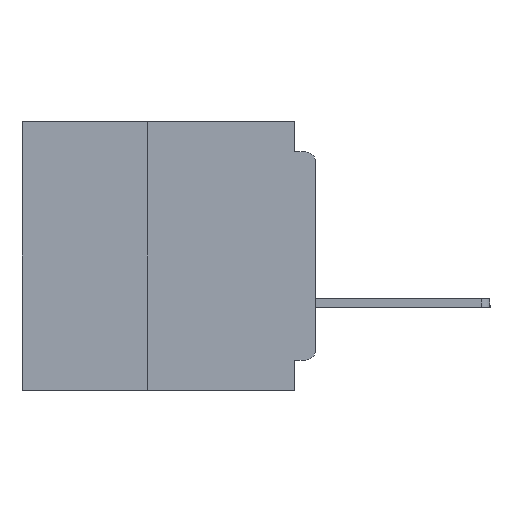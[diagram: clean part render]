
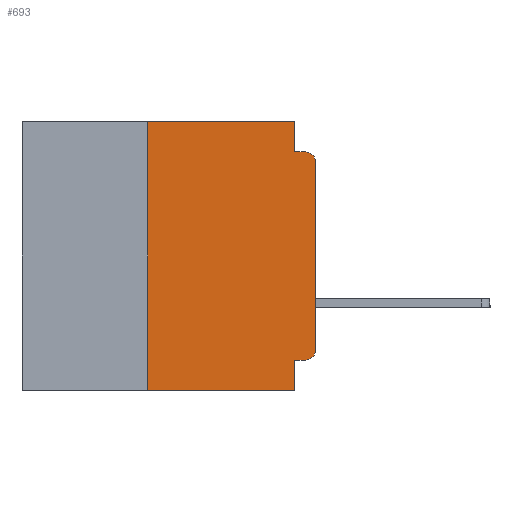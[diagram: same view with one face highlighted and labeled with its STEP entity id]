
A CAD part, left-side view. The second image highlights one B-rep face of the part: STEP entity #693.
In plain terms, the highlighted planar face has unit normal (-1, 0, 0).
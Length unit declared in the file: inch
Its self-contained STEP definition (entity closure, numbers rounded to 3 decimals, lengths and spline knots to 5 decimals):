
#657 = VERTEX_POINT ( 'NONE', #3051 ) ;
#693 = ADVANCED_FACE ( 'NONE', ( #32151 ), #5395, .F. ) ;
#718 = CARTESIAN_POINT ( 'NONE',  ( 0., 0.031, -0.045 ) ) ;
#1329 = DIRECTION ( 'NONE',  ( 0., -1., 0. ) ) ;
#1890 = CARTESIAN_POINT ( 'NONE',  ( 0., 0., -0.355 ) ) ;
#2554 = CARTESIAN_POINT ( 'NONE',  ( 0., 0.015, -0.355 ) ) ;
#3051 = CARTESIAN_POINT ( 'NONE',  ( 0., 0., -0.06 ) ) ;
#3372 = AXIS2_PLACEMENT_3D ( 'NONE', #11242, #6057, #5957 ) ;
#4143 = CARTESIAN_POINT ( 'NONE',  ( 0., 0.031, -0.4 ) ) ;
#4748 = DIRECTION ( 'NONE',  ( 0., -1., 0. ) ) ;
#4871 = VECTOR ( 'NONE', #12030, 39.37008 ) ;
#5310 = EDGE_LOOP ( 'NONE', ( #17593, #26373, #27103, #8839, #28532, #6120, #42472, #32633, #36755, #35333 ) ) ;
#5320 = DIRECTION ( 'NONE',  ( 0., 1., 0. ) ) ;
#5395 = PLANE ( 'NONE',  #3372 ) ;
#5957 = DIRECTION ( 'NONE',  ( 0., 0., -1. ) ) ;
#6057 = DIRECTION ( 'NONE',  ( 1., 0., 0. ) ) ;
#6120 = ORIENTED_EDGE ( 'NONE', *, *, #15140, .F. ) ;
#6469 = CARTESIAN_POINT ( 'NONE',  ( 0., 0.031, 0. ) ) ;
#6547 = VERTEX_POINT ( 'NONE', #18486 ) ;
#6554 = DIRECTION ( 'NONE',  ( 0., -1., 0. ) ) ;
#8559 = EDGE_CURVE ( 'NONE', #16307, #34333, #42617, .T. ) ;
#8569 = CARTESIAN_POINT ( 'NONE',  ( 0., 0.031, 0. ) ) ;
#8839 = ORIENTED_EDGE ( 'NONE', *, *, #38920, .F. ) ;
#9049 = DIRECTION ( 'NONE',  ( -1., 0., 0. ) ) ;
#9460 = VERTEX_POINT ( 'NONE', #6469 ) ;
#10446 = AXIS2_PLACEMENT_3D ( 'NONE', #29039, #9049, #32432 ) ;
#10729 = LINE ( 'NONE', #41371, #36214 ) ;
#11242 = CARTESIAN_POINT ( 'NONE',  ( 0., 0.437, 0. ) ) ;
#12005 = LINE ( 'NONE', #43093, #37463 ) ;
#12030 = DIRECTION ( 'NONE',  ( 0., 0., -1. ) ) ;
#13541 = DIRECTION ( 'NONE',  ( 0., 0., 1. ) ) ;
#13799 = LINE ( 'NONE', #14898, #21631 ) ;
#14363 = VERTEX_POINT ( 'NONE', #30455 ) ;
#14898 = CARTESIAN_POINT ( 'NONE',  ( 0., 0.437, 0. ) ) ;
#15065 = CIRCLE ( 'NONE', #33248, 0.015 ) ;
#15140 = EDGE_CURVE ( 'NONE', #6547, #39524, #37476, .T. ) ;
#16307 = VERTEX_POINT ( 'NONE', #2554 ) ;
#17262 = VERTEX_POINT ( 'NONE', #40918 ) ;
#17593 = ORIENTED_EDGE ( 'NONE', *, *, #25316, .T. ) ;
#18357 = CARTESIAN_POINT ( 'NONE',  ( 0., 0.25, -0.4 ) ) ;
#18486 = CARTESIAN_POINT ( 'NONE',  ( 0., 0.25, -0.4 ) ) ;
#18501 = EDGE_CURVE ( 'NONE', #39524, #9460, #13799, .T. ) ;
#18557 = VECTOR ( 'NONE', #13541, 39.37008 ) ;
#19744 = CARTESIAN_POINT ( 'NONE',  ( 0., 0.015, -0.06 ) ) ;
#21074 = EDGE_CURVE ( 'NONE', #42558, #14363, #10729, .T. ) ;
#21631 = VECTOR ( 'NONE', #1329, 39.37008 ) ;
#22502 = CARTESIAN_POINT ( 'NONE',  ( 0., 0.031, -0.355 ) ) ;
#23019 = VECTOR ( 'NONE', #5320, 39.37008 ) ;
#23118 = DIRECTION ( 'NONE',  ( 0., 0., -1. ) ) ;
#24790 = EDGE_CURVE ( 'NONE', #34333, #32093, #33334, .T. ) ;
#25316 = EDGE_CURVE ( 'NONE', #17262, #657, #26349, .T. ) ;
#26349 = LINE ( 'NONE', #36772, #18557 ) ;
#26373 = ORIENTED_EDGE ( 'NONE', *, *, #39118, .T. ) ;
#27103 = ORIENTED_EDGE ( 'NONE', *, *, #21074, .F. ) ;
#27257 = DIRECTION ( 'NONE',  ( 0., 0., -1. ) ) ;
#28532 = ORIENTED_EDGE ( 'NONE', *, *, #18501, .F. ) ;
#28661 = VECTOR ( 'NONE', #41493, 39.37008 ) ;
#29039 = CARTESIAN_POINT ( 'NONE',  ( 0., 0.015, -0.34 ) ) ;
#29772 = CIRCLE ( 'NONE', #10446, 0.015 ) ;
#30455 = CARTESIAN_POINT ( 'NONE',  ( 0., 0.015, -0.045 ) ) ;
#31625 = LINE ( 'NONE', #8569, #4871 ) ;
#32093 = VERTEX_POINT ( 'NONE', #4143 ) ;
#32151 = FACE_OUTER_BOUND ( 'NONE', #5310, .T. ) ;
#32361 = CARTESIAN_POINT ( 'NONE',  ( 0., 0.25, 0. ) ) ;
#32432 = DIRECTION ( 'NONE',  ( 0., 0., -1. ) ) ;
#32633 = ORIENTED_EDGE ( 'NONE', *, *, #24790, .F. ) ;
#33248 = AXIS2_PLACEMENT_3D ( 'NONE', #19744, #42861, #23118 ) ;
#33334 = LINE ( 'NONE', #33945, #42051 ) ;
#33337 = EDGE_CURVE ( 'NONE', #6547, #32093, #12005, .T. ) ;
#33945 = CARTESIAN_POINT ( 'NONE',  ( 0., 0.031, -0.4 ) ) ;
#34333 = VERTEX_POINT ( 'NONE', #22502 ) ;
#35333 = ORIENTED_EDGE ( 'NONE', *, *, #42803, .T. ) ;
#36214 = VECTOR ( 'NONE', #4748, 39.37008 ) ;
#36755 = ORIENTED_EDGE ( 'NONE', *, *, #8559, .F. ) ;
#36772 = CARTESIAN_POINT ( 'NONE',  ( 0., 0., 0. ) ) ;
#37463 = VECTOR ( 'NONE', #6554, 39.37008 ) ;
#37476 = LINE ( 'NONE', #18357, #28661 ) ;
#38920 = EDGE_CURVE ( 'NONE', #9460, #42558, #31625, .T. ) ;
#39118 = EDGE_CURVE ( 'NONE', #657, #14363, #15065, .T. ) ;
#39524 = VERTEX_POINT ( 'NONE', #32361 ) ;
#40918 = CARTESIAN_POINT ( 'NONE',  ( 0., 0., -0.34 ) ) ;
#41371 = CARTESIAN_POINT ( 'NONE',  ( 0., 0., -0.045 ) ) ;
#41493 = DIRECTION ( 'NONE',  ( 0., 0., 1. ) ) ;
#42051 = VECTOR ( 'NONE', #27257, 39.37008 ) ;
#42472 = ORIENTED_EDGE ( 'NONE', *, *, #33337, .T. ) ;
#42558 = VERTEX_POINT ( 'NONE', #718 ) ;
#42617 = LINE ( 'NONE', #1890, #23019 ) ;
#42803 = EDGE_CURVE ( 'NONE', #16307, #17262, #29772, .T. ) ;
#42861 = DIRECTION ( 'NONE',  ( -1., 0., 0. ) ) ;
#43093 = CARTESIAN_POINT ( 'NONE',  ( 0., 0.437, -0.4 ) ) ;
